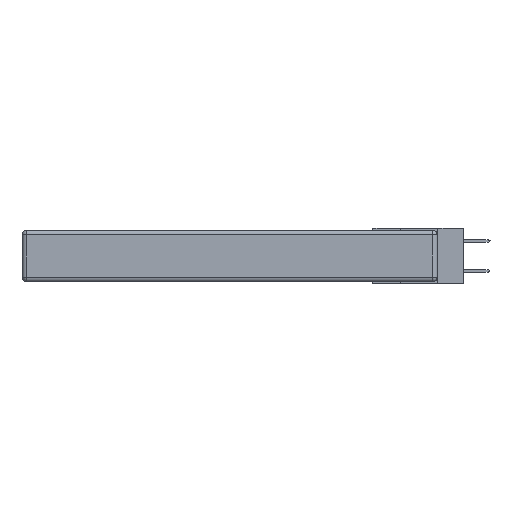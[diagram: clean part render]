
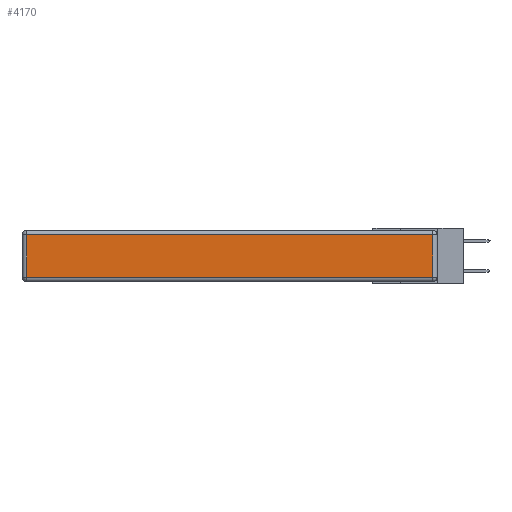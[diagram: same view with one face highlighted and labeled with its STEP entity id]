
A CAD part, left-side view. The second image highlights one B-rep face of the part: STEP entity #4170.
In plain terms, the highlighted planar face has unit normal (-1, 0, 0).
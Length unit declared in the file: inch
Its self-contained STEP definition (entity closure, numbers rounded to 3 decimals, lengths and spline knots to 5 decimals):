
#593 = VECTOR ( 'NONE', #19285, 39.37008 ) ;
#2251 = ORIENTED_EDGE ( 'NONE', *, *, #18306, .T. ) ;
#3504 = ORIENTED_EDGE ( 'NONE', *, *, #6098, .T. ) ;
#3775 = VECTOR ( 'NONE', #8140, 39.37008 ) ;
#4170 = ADVANCED_FACE ( 'NONE', ( #22586 ), #19644, .T. ) ;
#6098 = EDGE_CURVE ( 'NONE', #14313, #26328, #22789, .T. ) ;
#6927 = CARTESIAN_POINT ( 'NONE',  ( 0., 0., -0.343 ) ) ;
#7085 = CARTESIAN_POINT ( 'NONE',  ( 0., 2.72, -0.03 ) ) ;
#7291 = EDGE_LOOP ( 'NONE', ( #3504, #2251, #21174, #26945 ) ) ;
#7300 = EDGE_CURVE ( 'NONE', #26199, #14313, #20370, .T. ) ;
#7940 = LINE ( 'NONE', #14416, #25377 ) ;
#8064 = CARTESIAN_POINT ( 'NONE',  ( 0., 0.03, -0.313 ) ) ;
#8140 = DIRECTION ( 'NONE',  ( 0., 1., 0. ) ) ;
#8753 = CARTESIAN_POINT ( 'NONE',  ( 0., 0.03, -0.03 ) ) ;
#11446 = VECTOR ( 'NONE', #27717, 39.37008 ) ;
#13477 = DIRECTION ( 'NONE',  ( -1., 0., 0. ) ) ;
#13623 = EDGE_CURVE ( 'NONE', #20562, #26199, #27272, .T. ) ;
#14313 = VERTEX_POINT ( 'NONE', #23878 ) ;
#14416 = CARTESIAN_POINT ( 'NONE',  ( 0., 0.03, -0.343 ) ) ;
#15270 = CARTESIAN_POINT ( 'NONE',  ( 0., 2.72, -0.343 ) ) ;
#15503 = DIRECTION ( 'NONE',  ( 0., 0., 1. ) ) ;
#16551 = DIRECTION ( 'NONE',  ( 0., 0., 1. ) ) ;
#18306 = EDGE_CURVE ( 'NONE', #26328, #20562, #7940, .T. ) ;
#19285 = DIRECTION ( 'NONE',  ( 0., 0., -1. ) ) ;
#19644 = PLANE ( 'NONE',  #25733 ) ;
#20370 = LINE ( 'NONE', #15270, #593 ) ;
#20562 = VERTEX_POINT ( 'NONE', #8753 ) ;
#21174 = ORIENTED_EDGE ( 'NONE', *, *, #13623, .T. ) ;
#22586 = FACE_OUTER_BOUND ( 'NONE', #7291, .T. ) ;
#22789 = LINE ( 'NONE', #25166, #11446 ) ;
#23230 = CARTESIAN_POINT ( 'NONE',  ( 0., 2.75, -0.03 ) ) ;
#23878 = CARTESIAN_POINT ( 'NONE',  ( 0., 2.72, -0.313 ) ) ;
#25166 = CARTESIAN_POINT ( 'NONE',  ( 0., 0., -0.313 ) ) ;
#25377 = VECTOR ( 'NONE', #16551, 39.37008 ) ;
#25733 = AXIS2_PLACEMENT_3D ( 'NONE', #6927, #13477, #15503 ) ;
#26199 = VERTEX_POINT ( 'NONE', #7085 ) ;
#26328 = VERTEX_POINT ( 'NONE', #8064 ) ;
#26945 = ORIENTED_EDGE ( 'NONE', *, *, #7300, .T. ) ;
#27272 = LINE ( 'NONE', #23230, #3775 ) ;
#27717 = DIRECTION ( 'NONE',  ( 0., -1., 0. ) ) ;
